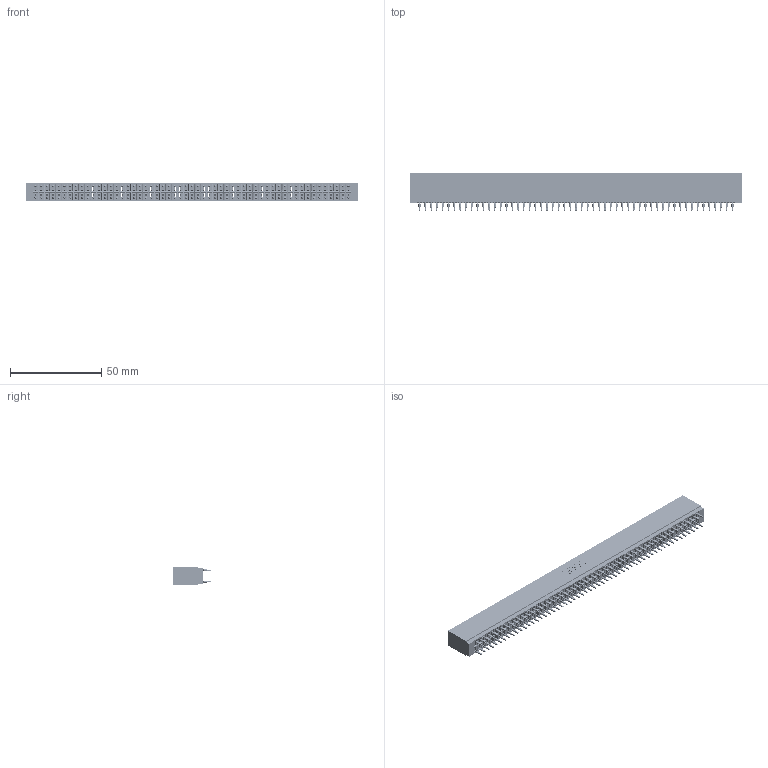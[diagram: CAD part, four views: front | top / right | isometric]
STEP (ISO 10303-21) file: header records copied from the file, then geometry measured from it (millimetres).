
FILE_DESCRIPTION (( 'STEP AP203' ), '1' );
FILE_NAME ('746-110-560-201.STEP', '2026-03-05T00:53:09', ( '' ), ( '' ), 'SwSTEP 2.0', 'SolidWorks 2023', '' );
FILE_SCHEMA (( 'CONFIG_CONTROL_DESIGN' ));
Length unit declared in the file: millimetre
Products named in the file (3): 746-110-560-201; 746-292-001_560; 746 Part_.515 Slot Depth - 01
Assembly tree (111 placements, depth 2):
  746-110-560-201
    746 Part_.515 Slot Depth - 01
    746-292-001_560  x110
Bounding box: 181.86 x 20.82 x 9.91 mm (x, y, z)
Volume: 19791.2 mm3; surface area: 33834.3 mm2
Topology: 111 solids, 111 shells, 10492 faces, 29193 edges, 18710 vertices
Faces by surface type: plane 5225, cylinder 2407, bspline 2200, torus 660
Entity records: 83226 total; most frequent: CARTESIAN_POINT 16429, ORIENTED_EDGE 14350, DIRECTION 11965, EDGE_CURVE 7175, VECTOR 6433, LINE 6433, VERTEX_POINT 4758, AXIS2_PLACEMENT_3D 2766
